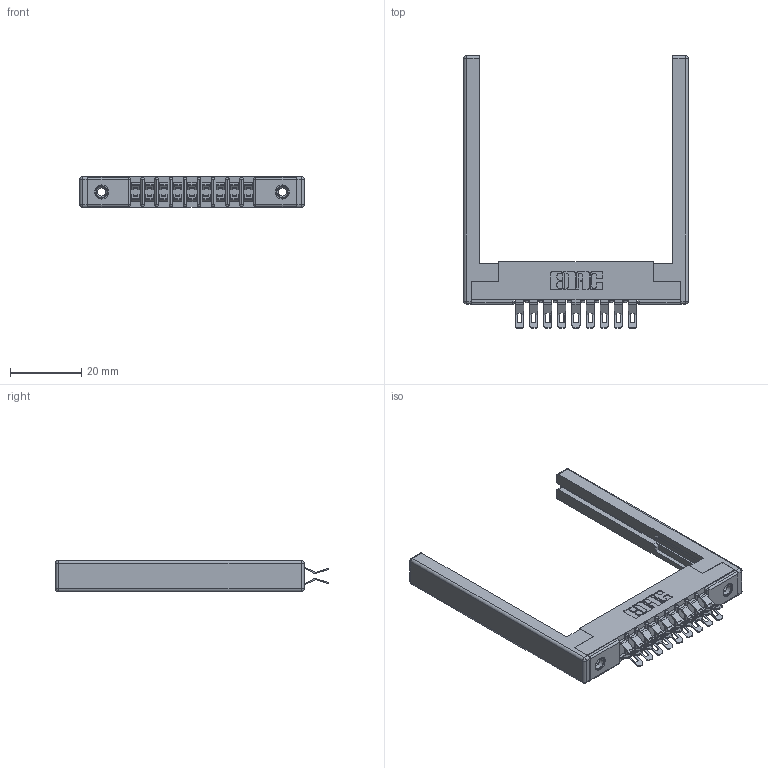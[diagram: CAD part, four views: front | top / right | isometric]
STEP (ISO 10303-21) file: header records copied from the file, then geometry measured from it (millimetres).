
FILE_DESCRIPTION (( 'STEP AP203' ), '1' );
FILE_NAME ('357-018-455-268.STEP', '2020-10-02T20:49:01', ( '' ), ( '' ), 'SwSTEP 2.0', 'SolidWorks 2020', '' );
FILE_SCHEMA (( 'CONFIG_CONTROL_DESIGN' ));
Length unit declared in the file: inch
Products named in the file (5): 307-220-068; 307 Part_.156 Dia Mounting Holes; 357-018-455-268; 345-250-001_345-250-001-102; 307-290-001_555
Assembly tree (23 placements, depth 2):
  357-018-455-268
    307 Part_.156 Dia Mounting Holes
    307-290-001_555  x18
    307-220-068  x2
    345-250-001_345-250-001-102  x2
Bounding box: 63.09 x 76.71 x 8.71 mm (x, y, z)
Volume: 8743.6 mm3; surface area: 11048.8 mm2
Topology: 23 solids, 23 shells, 1380 faces, 3971 edges, 2574 vertices
Faces by surface type: plane 770, cylinder 566, sphere 28, cone 12, torus 4
Entity records: 15368 total; most frequent: CARTESIAN_POINT 2506, DIRECTION 2491, ORIENTED_EDGE 2474, EDGE_CURVE 1237, LINE 921, VECTOR 921, VERTEX_POINT 800, AXIS2_PLACEMENT_3D 785
